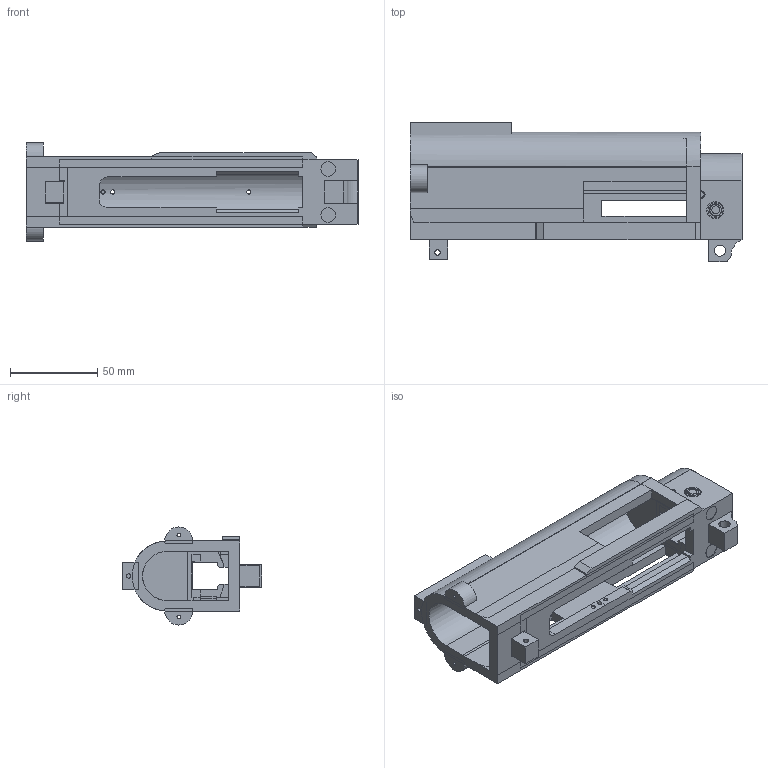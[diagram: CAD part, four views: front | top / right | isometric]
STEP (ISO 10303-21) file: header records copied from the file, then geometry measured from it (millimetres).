
FILE_DESCRIPTION(('FreeCAD Model'),'2;1');
FILE_NAME('AP9upper.step', '2017-11-13T22:54:48',('Author'),(''), 'Open CASCADE STEP processor 6.8','FreeCAD','Unknown');
FILE_SCHEMA(('AUTOMOTIVE_DESIGN_CC2 { 1 2 10303 214 -1 1 5 4 }'));
Length unit declared in the file: millimetre
Products named in the file (1): Pocket013
Bounding box: 190.38 x 80.21 x 56.2 mm (x, y, z)
Volume: 188423.5 mm3; surface area: 63935.8 mm2
Topology: 1 solids, 2 shells, 286 faces, 834 edges, 560 vertices
Faces by surface type: plane 240, cylinder 46
Full cylindrical faces by diameter (mm): 2 x3, 2.4 x12, 8 x1, 8.4 x2
Entity records: 23523 total; most frequent: CARTESIAN_POINT 7329, DIRECTION 2872, LINE 1940, VECTOR 1940, ORIENTED_EDGE 1668, PCURVE 1668, DEFINITIONAL_REPRESENTATION 1668, EDGE_CURVE 834
